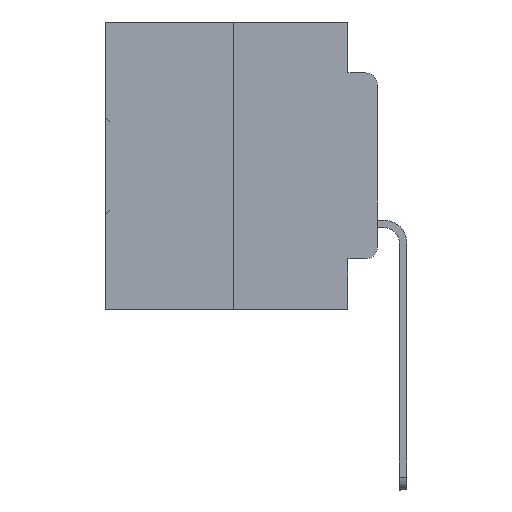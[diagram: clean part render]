
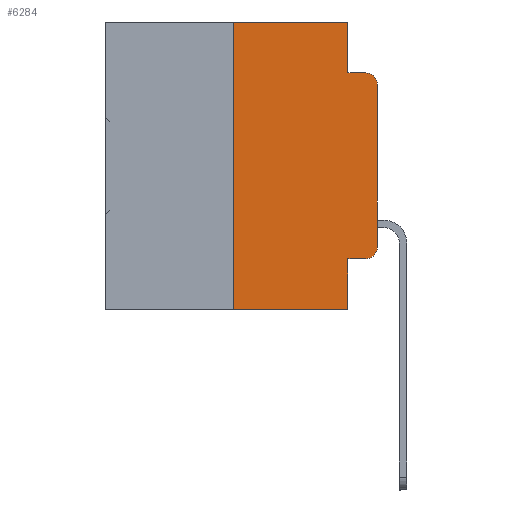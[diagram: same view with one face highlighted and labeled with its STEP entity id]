
A CAD part, left-side view. The second image highlights one B-rep face of the part: STEP entity #6284.
In plain terms, the highlighted planar face has unit normal (-1, 0, 0).
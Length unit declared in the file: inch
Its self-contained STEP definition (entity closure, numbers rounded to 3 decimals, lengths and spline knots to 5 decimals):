
#1607 = LINE ( 'NONE', #7509, #15506 ) ;
#1876 = VECTOR ( 'NONE', #24054, 39.37008 ) ;
#2089 = CARTESIAN_POINT ( 'NONE',  ( 0., 0.051, 0. ) ) ;
#2109 = LINE ( 'NONE', #31978, #23170 ) ;
#2435 = DIRECTION ( 'NONE',  ( 0., 0., -1. ) ) ;
#2488 = CARTESIAN_POINT ( 'NONE',  ( 0., 0.051, -0.4115 ) ) ;
#2709 = VERTEX_POINT ( 'NONE', #4004 ) ;
#2855 = DIRECTION ( 'NONE',  ( 0., 0., -1. ) ) ;
#3053 = VECTOR ( 'NONE', #16628, 39.37008 ) ;
#3801 = CARTESIAN_POINT ( 'NONE',  ( 0., 0.051, 0. ) ) ;
#4004 = CARTESIAN_POINT ( 'NONE',  ( 0., 0.25, -0.5 ) ) ;
#4722 = CARTESIAN_POINT ( 'NONE',  ( 0., 0.051, -0.4115 ) ) ;
#5327 = DIRECTION ( 'NONE',  ( 0., -1., 0. ) ) ;
#5777 = CARTESIAN_POINT ( 'NONE',  ( 0., 0., -0.3915 ) ) ;
#5867 = VECTOR ( 'NONE', #5327, 39.37008 ) ;
#6273 = VERTEX_POINT ( 'NONE', #8876 ) ;
#6284 = ADVANCED_FACE ( 'NONE', ( #16041 ), #17011, .F. ) ;
#6922 = EDGE_CURVE ( 'NONE', #20319, #10856, #33188, .T. ) ;
#7509 = CARTESIAN_POINT ( 'NONE',  ( 0., 0., 0. ) ) ;
#8368 = CARTESIAN_POINT ( 'NONE',  ( 0., 0.473, 0. ) ) ;
#8717 = CARTESIAN_POINT ( 'NONE',  ( 0., 0.02, -0.3915 ) ) ;
#8876 = CARTESIAN_POINT ( 'NONE',  ( 0., 0.051, -0.0885 ) ) ;
#10856 = VERTEX_POINT ( 'NONE', #5777 ) ;
#10907 = ORIENTED_EDGE ( 'NONE', *, *, #18882, .F. ) ;
#10924 = CARTESIAN_POINT ( 'NONE',  ( 0., 0.051, -0.0885 ) ) ;
#11499 = DIRECTION ( 'NONE',  ( 0., 0., -1. ) ) ;
#11697 = CARTESIAN_POINT ( 'NONE',  ( 0., 0.02, -0.4115 ) ) ;
#11728 = ORIENTED_EDGE ( 'NONE', *, *, #23629, .T. ) ;
#11993 = VECTOR ( 'NONE', #2855, 39.37008 ) ;
#13376 = ORIENTED_EDGE ( 'NONE', *, *, #31867, .T. ) ;
#13454 = AXIS2_PLACEMENT_3D ( 'NONE', #27855, #33159, #17135 ) ;
#14994 = EDGE_CURVE ( 'NONE', #2709, #28675, #2109, .T. ) ;
#15093 = VECTOR ( 'NONE', #18435, 39.37008 ) ;
#15153 = LINE ( 'NONE', #16245, #34788 ) ;
#15455 = EDGE_CURVE ( 'NONE', #28827, #20319, #29407, .T. ) ;
#15506 = VECTOR ( 'NONE', #31944, 39.37008 ) ;
#16041 = FACE_OUTER_BOUND ( 'NONE', #21563, .T. ) ;
#16245 = CARTESIAN_POINT ( 'NONE',  ( 0., 0.25, 0. ) ) ;
#16618 = CARTESIAN_POINT ( 'NONE',  ( 0., 0.051, 0. ) ) ;
#16628 = DIRECTION ( 'NONE',  ( 0., -1., 0. ) ) ;
#16736 = CARTESIAN_POINT ( 'NONE',  ( 0., 0.25, 0. ) ) ;
#16761 = VERTEX_POINT ( 'NONE', #21404 ) ;
#17011 = PLANE ( 'NONE',  #13454 ) ;
#17135 = DIRECTION ( 'NONE',  ( 0., 0., -1. ) ) ;
#17393 = ORIENTED_EDGE ( 'NONE', *, *, #6922, .T. ) ;
#18358 = LINE ( 'NONE', #16618, #11993 ) ;
#18430 = EDGE_CURVE ( 'NONE', #28827, #28675, #18358, .T. ) ;
#18435 = DIRECTION ( 'NONE',  ( 0., -1., 0. ) ) ;
#18470 = VERTEX_POINT ( 'NONE', #16736 ) ;
#18882 = EDGE_CURVE ( 'NONE', #21683, #6273, #23797, .T. ) ;
#18951 = DIRECTION ( 'NONE',  ( -1., 0., 0. ) ) ;
#18972 = DIRECTION ( 'NONE',  ( 0., 0., 1. ) ) ;
#20319 = VERTEX_POINT ( 'NONE', #11697 ) ;
#20354 = ORIENTED_EDGE ( 'NONE', *, *, #24307, .F. ) ;
#20439 = LINE ( 'NONE', #10924, #5867 ) ;
#20803 = EDGE_CURVE ( 'NONE', #18470, #21683, #24907, .T. ) ;
#21363 = EDGE_CURVE ( 'NONE', #2709, #18470, #15153, .T. ) ;
#21394 = DIRECTION ( 'NONE',  ( 0., -1., 0. ) ) ;
#21404 = CARTESIAN_POINT ( 'NONE',  ( 0., 0., -0.1085 ) ) ;
#21563 = EDGE_LOOP ( 'NONE', ( #13376, #11728, #20354, #10907, #24584, #25051, #25727, #27358, #27688, #17393 ) ) ;
#21683 = VERTEX_POINT ( 'NONE', #3801 ) ;
#23170 = VECTOR ( 'NONE', #21394, 39.37008 ) ;
#23256 = CARTESIAN_POINT ( 'NONE',  ( 0., 0.02, -0.0885 ) ) ;
#23629 = EDGE_CURVE ( 'NONE', #16761, #27528, #28889, .T. ) ;
#23797 = LINE ( 'NONE', #2089, #1876 ) ;
#24054 = DIRECTION ( 'NONE',  ( 0., 0., -1. ) ) ;
#24307 = EDGE_CURVE ( 'NONE', #6273, #27528, #20439, .T. ) ;
#24584 = ORIENTED_EDGE ( 'NONE', *, *, #20803, .F. ) ;
#24907 = LINE ( 'NONE', #8368, #3053 ) ;
#25051 = ORIENTED_EDGE ( 'NONE', *, *, #21363, .F. ) ;
#25727 = ORIENTED_EDGE ( 'NONE', *, *, #14994, .T. ) ;
#27358 = ORIENTED_EDGE ( 'NONE', *, *, #18430, .F. ) ;
#27528 = VERTEX_POINT ( 'NONE', #23256 ) ;
#27688 = ORIENTED_EDGE ( 'NONE', *, *, #15455, .T. ) ;
#27712 = DIRECTION ( 'NONE',  ( -1., 0., 0. ) ) ;
#27855 = CARTESIAN_POINT ( 'NONE',  ( 0., 0.473, 0. ) ) ;
#28675 = VERTEX_POINT ( 'NONE', #28984 ) ;
#28827 = VERTEX_POINT ( 'NONE', #2488 ) ;
#28889 = CIRCLE ( 'NONE', #33919, 0.02 ) ;
#28984 = CARTESIAN_POINT ( 'NONE',  ( 0., 0.051, -0.5 ) ) ;
#29018 = AXIS2_PLACEMENT_3D ( 'NONE', #8717, #27712, #11499 ) ;
#29407 = LINE ( 'NONE', #4722, #15093 ) ;
#31867 = EDGE_CURVE ( 'NONE', #10856, #16761, #1607, .T. ) ;
#31944 = DIRECTION ( 'NONE',  ( 0., 0., 1. ) ) ;
#31978 = CARTESIAN_POINT ( 'NONE',  ( 0., 0.473, -0.5 ) ) ;
#33159 = DIRECTION ( 'NONE',  ( 1., 0., 0. ) ) ;
#33188 = CIRCLE ( 'NONE', #29018, 0.02 ) ;
#33919 = AXIS2_PLACEMENT_3D ( 'NONE', #34883, #18951, #2435 ) ;
#34788 = VECTOR ( 'NONE', #18972, 39.37008 ) ;
#34883 = CARTESIAN_POINT ( 'NONE',  ( 0., 0.02, -0.1085 ) ) ;
